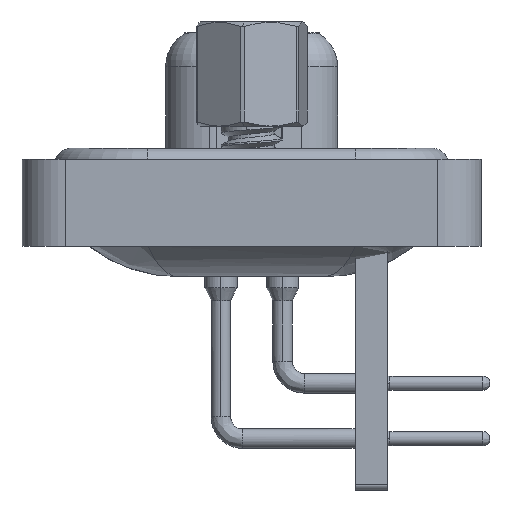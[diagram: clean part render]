
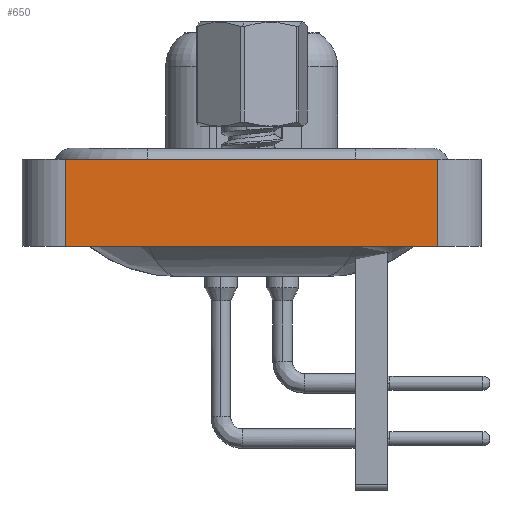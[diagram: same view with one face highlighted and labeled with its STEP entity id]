
A CAD part, left-side view. The second image highlights one B-rep face of the part: STEP entity #650.
In plain terms, the highlighted planar face has unit normal (-1, 0, 0).
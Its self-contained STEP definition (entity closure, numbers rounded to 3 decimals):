
#650 = ADVANCED_FACE ( 'NONE', ( #18071 ), #10681, .T. ) ;
#946 = DIRECTION ( 'NONE',  ( 0., 0., 1. ) ) ;
#1855 = EDGE_CURVE ( 'NONE', #14512, #14876, #9866, .T. ) ;
#2014 = ORIENTED_EDGE ( 'NONE', *, *, #1855, .T. ) ;
#2290 = EDGE_CURVE ( 'NONE', #8911, #5277, #10630, .T. ) ;
#3891 = VECTOR ( 'NONE', #4133, 1000. ) ;
#4133 = DIRECTION ( 'NONE',  ( 0., 0., 1. ) ) ;
#5277 = VERTEX_POINT ( 'NONE', #12888 ) ;
#5446 = VECTOR ( 'NONE', #21870, 1000. ) ;
#6215 = CARTESIAN_POINT ( 'NONE',  ( -7.285, -8.55, -3.6 ) ) ;
#6238 = ORIENTED_EDGE ( 'NONE', *, *, #2290, .F. ) ;
#7327 = EDGE_CURVE ( 'NONE', #8911, #14512, #14583, .T. ) ;
#8911 = VERTEX_POINT ( 'NONE', #24350 ) ;
#9443 = VECTOR ( 'NONE', #14329, 1000. ) ;
#9492 = CARTESIAN_POINT ( 'NONE',  ( -7.285, -8.55, -3.6 ) ) ;
#9866 = LINE ( 'NONE', #9492, #3891 ) ;
#9915 = ORIENTED_EDGE ( 'NONE', *, *, #7327, .T. ) ;
#10630 = LINE ( 'NONE', #24772, #12407 ) ;
#10681 = PLANE ( 'NONE',  #16459 ) ;
#11908 = CARTESIAN_POINT ( 'NONE',  ( -7.285, -8.55, 0.4 ) ) ;
#12407 = VECTOR ( 'NONE', #946, 1000. ) ;
#12888 = CARTESIAN_POINT ( 'NONE',  ( -7.285, 8.55, 0.4 ) ) ;
#13476 = CARTESIAN_POINT ( 'NONE',  ( -7.285, -8.55, 0.4 ) ) ;
#14136 = DIRECTION ( 'NONE',  ( 0., 0., 1. ) ) ;
#14329 = DIRECTION ( 'NONE',  ( 0., -1., 0. ) ) ;
#14512 = VERTEX_POINT ( 'NONE', #6215 ) ;
#14583 = LINE ( 'NONE', #20333, #9443 ) ;
#14876 = VERTEX_POINT ( 'NONE', #13476 ) ;
#15855 = LINE ( 'NONE', #11908, #5446 ) ;
#16407 = CARTESIAN_POINT ( 'NONE',  ( -7.285, -8.55, -3.6 ) ) ;
#16459 = AXIS2_PLACEMENT_3D ( 'NONE', #16407, #18458, #14136 ) ;
#17148 = EDGE_CURVE ( 'NONE', #5277, #14876, #15855, .T. ) ;
#18071 = FACE_OUTER_BOUND ( 'NONE', #23900, .T. ) ;
#18458 = DIRECTION ( 'NONE',  ( -1., 0., 0. ) ) ;
#18981 = ORIENTED_EDGE ( 'NONE', *, *, #17148, .F. ) ;
#20333 = CARTESIAN_POINT ( 'NONE',  ( -7.285, -8.55, -3.6 ) ) ;
#21870 = DIRECTION ( 'NONE',  ( 0., -1., 0. ) ) ;
#23900 = EDGE_LOOP ( 'NONE', ( #2014, #18981, #6238, #9915 ) ) ;
#24350 = CARTESIAN_POINT ( 'NONE',  ( -7.285, 8.55, -3.6 ) ) ;
#24772 = CARTESIAN_POINT ( 'NONE',  ( -7.285, 8.55, -3.6 ) ) ;
